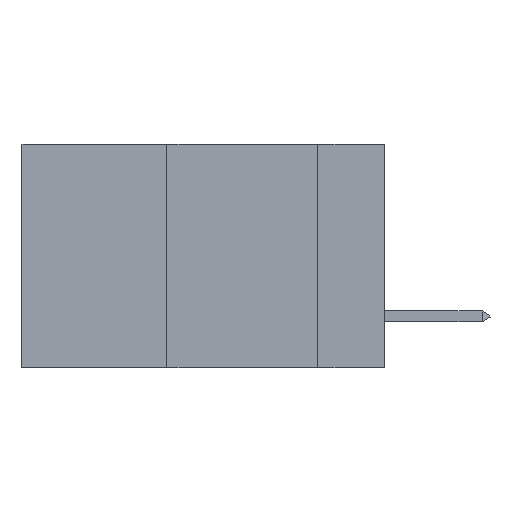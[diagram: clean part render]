
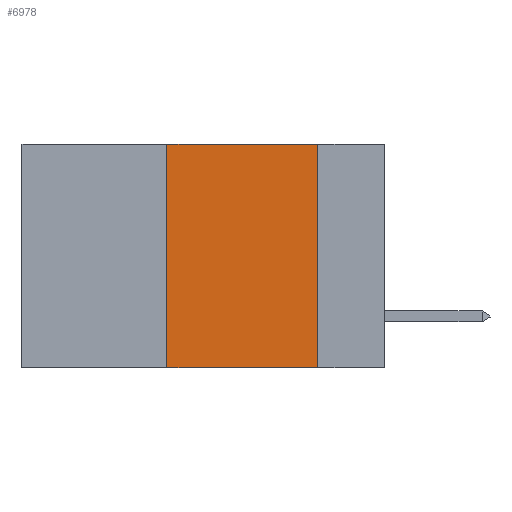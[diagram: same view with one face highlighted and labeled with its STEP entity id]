
A CAD part, left-side view. The second image highlights one B-rep face of the part: STEP entity #6978.
In plain terms, the highlighted planar face has unit normal (-1, 0, 0).
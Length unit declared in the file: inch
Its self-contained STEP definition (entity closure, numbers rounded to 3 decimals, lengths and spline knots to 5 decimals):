
#3963 = VERTEX_POINT ( 'NONE', #33728 ) ;
#6978 = ADVANCED_FACE ( 'NONE', ( #9585 ), #18620, .F. ) ;
#7120 = CARTESIAN_POINT ( 'NONE',  ( 0., 0.6, 0. ) ) ;
#7739 = ORIENTED_EDGE ( 'NONE', *, *, #43004, .F. ) ;
#9176 = LINE ( 'NONE', #29218, #21549 ) ;
#9585 = FACE_OUTER_BOUND ( 'NONE', #10775, .T. ) ;
#9816 = LINE ( 'NONE', #16671, #17852 ) ;
#10775 = EDGE_LOOP ( 'NONE', ( #41901, #7739, #14875, #38258 ) ) ;
#12155 = CARTESIAN_POINT ( 'NONE',  ( 0., 0.36, 0. ) ) ;
#14326 = EDGE_CURVE ( 'NONE', #3963, #30309, #9816, .T. ) ;
#14875 = ORIENTED_EDGE ( 'NONE', *, *, #33996, .F. ) ;
#14986 = DIRECTION ( 'NONE',  ( 0., 0., -1. ) ) ;
#16671 = CARTESIAN_POINT ( 'NONE',  ( 0., 0.6, -0.37 ) ) ;
#17852 = VECTOR ( 'NONE', #34174, 39.37008 ) ;
#18015 = DIRECTION ( 'NONE',  ( 0., -1., 0. ) ) ;
#18620 = PLANE ( 'NONE',  #41300 ) ;
#18839 = DIRECTION ( 'NONE',  ( 0., 0., 1. ) ) ;
#19288 = VERTEX_POINT ( 'NONE', #12155 ) ;
#20301 = VERTEX_POINT ( 'NONE', #21940 ) ;
#20641 = VECTOR ( 'NONE', #18015, 39.37008 ) ;
#21549 = VECTOR ( 'NONE', #18839, 39.37008 ) ;
#21940 = CARTESIAN_POINT ( 'NONE',  ( 0., 0.11, 0. ) ) ;
#29218 = CARTESIAN_POINT ( 'NONE',  ( 0., 0.36, 0. ) ) ;
#29485 = LINE ( 'NONE', #36682, #38126 ) ;
#30309 = VERTEX_POINT ( 'NONE', #36451 ) ;
#33728 = CARTESIAN_POINT ( 'NONE',  ( 0., 0.36, -0.37 ) ) ;
#33996 = EDGE_CURVE ( 'NONE', #3963, #19288, #9176, .T. ) ;
#34174 = DIRECTION ( 'NONE',  ( 0., -1., 0. ) ) ;
#36181 = EDGE_CURVE ( 'NONE', #20301, #30309, #29485, .T. ) ;
#36451 = CARTESIAN_POINT ( 'NONE',  ( 0., 0.11, -0.37 ) ) ;
#36682 = CARTESIAN_POINT ( 'NONE',  ( 0., 0.11, 0. ) ) ;
#38126 = VECTOR ( 'NONE', #44615, 39.37008 ) ;
#38258 = ORIENTED_EDGE ( 'NONE', *, *, #14326, .T. ) ;
#39468 = DIRECTION ( 'NONE',  ( 1., 0., 0. ) ) ;
#41300 = AXIS2_PLACEMENT_3D ( 'NONE', #42929, #39468, #14986 ) ;
#41901 = ORIENTED_EDGE ( 'NONE', *, *, #36181, .F. ) ;
#42929 = CARTESIAN_POINT ( 'NONE',  ( 0., 0.6, 0. ) ) ;
#43004 = EDGE_CURVE ( 'NONE', #19288, #20301, #43334, .T. ) ;
#43334 = LINE ( 'NONE', #7120, #20641 ) ;
#44615 = DIRECTION ( 'NONE',  ( 0., 0., -1. ) ) ;
